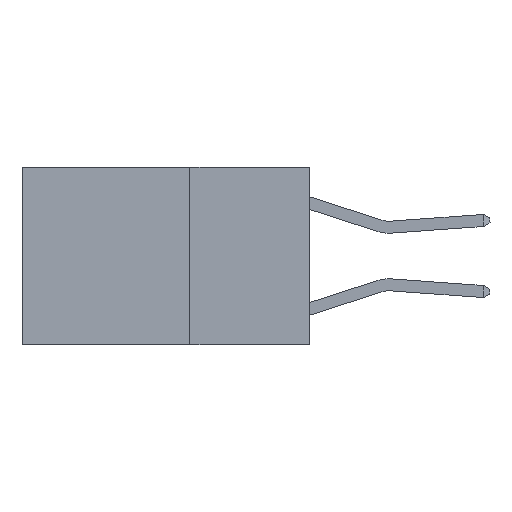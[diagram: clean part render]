
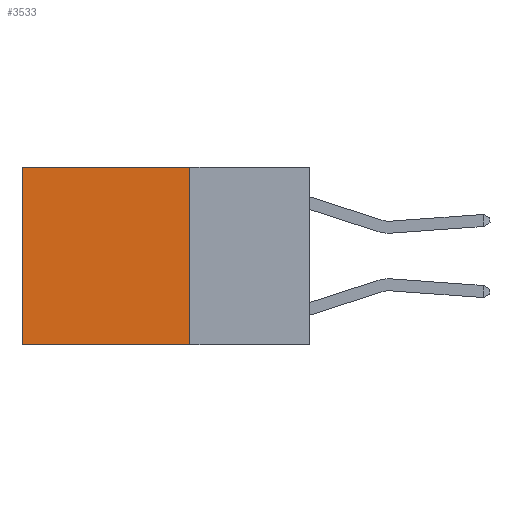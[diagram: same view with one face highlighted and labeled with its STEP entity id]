
A CAD part, left-side view. The second image highlights one B-rep face of the part: STEP entity #3533.
In plain terms, the highlighted planar face has unit normal (-1, 0, 0).
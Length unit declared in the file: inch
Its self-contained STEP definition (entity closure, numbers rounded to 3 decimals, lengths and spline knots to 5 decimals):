
#16 = ORIENTED_EDGE ( 'NONE', *, *, #8137, .T. ) ;
#248 = CARTESIAN_POINT ( 'NONE',  ( 0.2625, 0.6, 0. ) ) ;
#696 = LINE ( 'NONE', #248, #9116 ) ;
#726 = VECTOR ( 'NONE', #7474, 39.37008 ) ;
#1304 = VERTEX_POINT ( 'NONE', #10511 ) ;
#1617 = VERTEX_POINT ( 'NONE', #9437 ) ;
#1809 = LINE ( 'NONE', #7822, #7545 ) ;
#2275 = CARTESIAN_POINT ( 'NONE',  ( 0.2625, 0.6, -0.37 ) ) ;
#2426 = VERTEX_POINT ( 'NONE', #6278 ) ;
#3016 = VECTOR ( 'NONE', #9830, 39.37008 ) ;
#3158 = DIRECTION ( 'NONE',  ( 1., 0., 0. ) ) ;
#3255 = CARTESIAN_POINT ( 'NONE',  ( 0.2625, 0.25, -0.37 ) ) ;
#3533 = ADVANCED_FACE ( 'NONE', ( #9552 ), #6322, .F. ) ;
#3750 = DIRECTION ( 'NONE',  ( 0., 1., 0. ) ) ;
#3971 = EDGE_CURVE ( 'NONE', #1617, #2426, #5189, .T. ) ;
#4235 = EDGE_CURVE ( 'NONE', #2426, #8041, #5057, .T. ) ;
#5057 = LINE ( 'NONE', #3255, #726 ) ;
#5189 = LINE ( 'NONE', #9803, #3016 ) ;
#5411 = ORIENTED_EDGE ( 'NONE', *, *, #3971, .F. ) ;
#5573 = EDGE_CURVE ( 'NONE', #1304, #8041, #696, .T. ) ;
#6278 = CARTESIAN_POINT ( 'NONE',  ( 0.2625, 0.25, -0.37 ) ) ;
#6322 = PLANE ( 'NONE',  #7315 ) ;
#7315 = AXIS2_PLACEMENT_3D ( 'NONE', #9634, #3158, #8424 ) ;
#7474 = DIRECTION ( 'NONE',  ( 0., 1., 0. ) ) ;
#7545 = VECTOR ( 'NONE', #3750, 39.37008 ) ;
#7822 = CARTESIAN_POINT ( 'NONE',  ( 0.2625, 0.25, 0. ) ) ;
#8041 = VERTEX_POINT ( 'NONE', #2275 ) ;
#8089 = EDGE_LOOP ( 'NONE', ( #9902, #9192, #5411, #16 ) ) ;
#8137 = EDGE_CURVE ( 'NONE', #1617, #1304, #1809, .T. ) ;
#8424 = DIRECTION ( 'NONE',  ( 0., 0., -1. ) ) ;
#9116 = VECTOR ( 'NONE', #9255, 39.37008 ) ;
#9192 = ORIENTED_EDGE ( 'NONE', *, *, #4235, .F. ) ;
#9255 = DIRECTION ( 'NONE',  ( 0., 0., -1. ) ) ;
#9437 = CARTESIAN_POINT ( 'NONE',  ( 0.2625, 0.25, 0. ) ) ;
#9552 = FACE_OUTER_BOUND ( 'NONE', #8089, .T. ) ;
#9634 = CARTESIAN_POINT ( 'NONE',  ( 0.2625, 0.25, 0. ) ) ;
#9803 = CARTESIAN_POINT ( 'NONE',  ( 0.2625, 0.25, 0. ) ) ;
#9830 = DIRECTION ( 'NONE',  ( 0., 0., -1. ) ) ;
#9902 = ORIENTED_EDGE ( 'NONE', *, *, #5573, .T. ) ;
#10511 = CARTESIAN_POINT ( 'NONE',  ( 0.2625, 0.6, 0. ) ) ;
